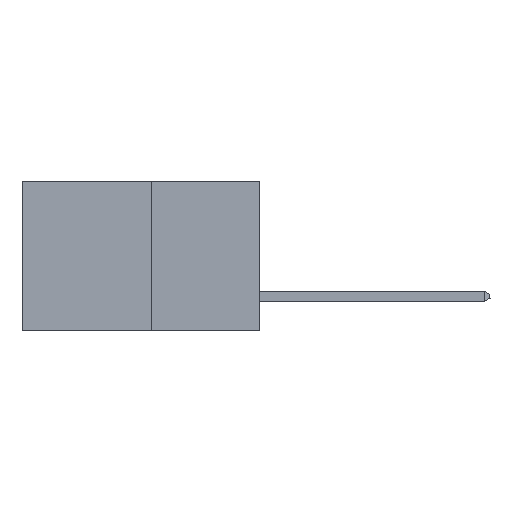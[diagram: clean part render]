
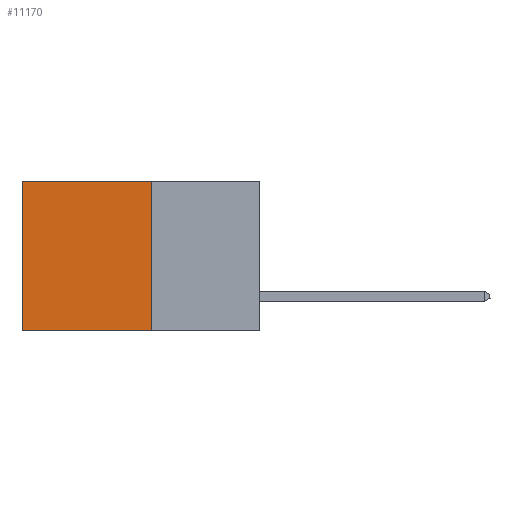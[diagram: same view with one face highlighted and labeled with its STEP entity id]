
A CAD part, left-side view. The second image highlights one B-rep face of the part: STEP entity #11170.
In plain terms, the highlighted planar face has unit normal (-1, 0, 0).
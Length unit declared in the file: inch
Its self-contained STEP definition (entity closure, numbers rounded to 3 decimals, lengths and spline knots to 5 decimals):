
#1450 = EDGE_CURVE ( 'NONE', #6504, #12572, #22794, .T. ) ;
#1706 = DIRECTION ( 'NONE',  ( 0., 0., -1. ) ) ;
#1922 = ORIENTED_EDGE ( 'NONE', *, *, #9079, .T. ) ;
#3816 = DIRECTION ( 'NONE',  ( 1., 0., 0. ) ) ;
#3831 = CARTESIAN_POINT ( 'NONE',  ( 0.277, 0.27, -0.37 ) ) ;
#5042 = LINE ( 'NONE', #10405, #18175 ) ;
#5894 = EDGE_LOOP ( 'NONE', ( #15039, #15802, #6599, #1922 ) ) ;
#6492 = DIRECTION ( 'NONE',  ( 0., 1., 0. ) ) ;
#6504 = VERTEX_POINT ( 'NONE', #16557 ) ;
#6599 = ORIENTED_EDGE ( 'NONE', *, *, #1450, .F. ) ;
#7398 = AXIS2_PLACEMENT_3D ( 'NONE', #15580, #3816, #17512 ) ;
#7429 = CARTESIAN_POINT ( 'NONE',  ( 0.277, 0.27, -0.37 ) ) ;
#7724 = PLANE ( 'NONE',  #7398 ) ;
#9079 = EDGE_CURVE ( 'NONE', #6504, #24298, #19310, .T. ) ;
#10405 = CARTESIAN_POINT ( 'NONE',  ( 0.277, 0.27, -0.37 ) ) ;
#11170 = ADVANCED_FACE ( 'NONE', ( #25224 ), #7724, .F. ) ;
#12572 = VERTEX_POINT ( 'NONE', #7429 ) ;
#13737 = VECTOR ( 'NONE', #1706, 39.37008 ) ;
#14020 = VECTOR ( 'NONE', #14545, 39.37008 ) ;
#14459 = CARTESIAN_POINT ( 'NONE',  ( 0.277, 0.59, -0.37 ) ) ;
#14545 = DIRECTION ( 'NONE',  ( 0., 0., -1. ) ) ;
#15039 = ORIENTED_EDGE ( 'NONE', *, *, #23521, .T. ) ;
#15580 = CARTESIAN_POINT ( 'NONE',  ( 0.277, 0.27, -0.37 ) ) ;
#15802 = ORIENTED_EDGE ( 'NONE', *, *, #25213, .F. ) ;
#16557 = CARTESIAN_POINT ( 'NONE',  ( 0.277, 0.27, 0. ) ) ;
#17512 = DIRECTION ( 'NONE',  ( 0., 0., -1. ) ) ;
#18175 = VECTOR ( 'NONE', #6492, 39.37008 ) ;
#19168 = LINE ( 'NONE', #14459, #14020 ) ;
#19310 = LINE ( 'NONE', #22765, #22629 ) ;
#21121 = CARTESIAN_POINT ( 'NONE',  ( 0.277, 0.59, 0. ) ) ;
#22461 = CARTESIAN_POINT ( 'NONE',  ( 0.277, 0.59, -0.37 ) ) ;
#22629 = VECTOR ( 'NONE', #24672, 39.37008 ) ;
#22765 = CARTESIAN_POINT ( 'NONE',  ( 0.277, 0.27, 0. ) ) ;
#22794 = LINE ( 'NONE', #3831, #13737 ) ;
#23521 = EDGE_CURVE ( 'NONE', #24298, #24124, #19168, .T. ) ;
#24124 = VERTEX_POINT ( 'NONE', #22461 ) ;
#24298 = VERTEX_POINT ( 'NONE', #21121 ) ;
#24672 = DIRECTION ( 'NONE',  ( 0., 1., 0. ) ) ;
#25213 = EDGE_CURVE ( 'NONE', #12572, #24124, #5042, .T. ) ;
#25224 = FACE_OUTER_BOUND ( 'NONE', #5894, .T. ) ;
